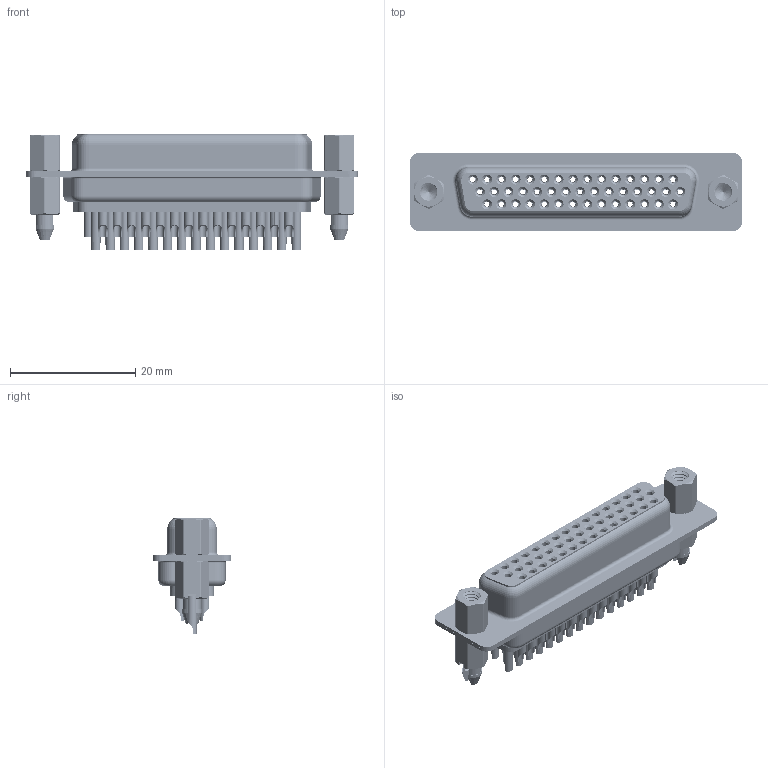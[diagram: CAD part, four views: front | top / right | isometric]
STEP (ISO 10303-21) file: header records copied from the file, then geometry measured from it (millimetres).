
FILE_DESCRIPTION (( 'STEP AP203' ), '1' );
FILE_NAME ('638-044-232-247.STEP', '2020-07-18T22:45:11', ( '' ), ( '' ), 'SwSTEP 2.0', 'SolidWorks 2020', '' );
FILE_SCHEMA (( 'CONFIG_CONTROL_DESIGN' ));
Length unit declared in the file: millimetre
Products named in the file (9): 638-044-232-247; 638 Shell Rear_44 Contacts; 638 Contact Row 1_32; 638 Shell Front_44 Contacts; 638 Contact Row 3_32; 638 Contact Row 2_32; 638 4-40 Threaded Boardlock_LP; 638 Housing_44 Contacts; 638 4-40 Hex Standoff
Assembly tree (51 placements, depth 2):
  638-044-232-247
    638 Housing_44 Contacts
    638 Shell Front_44 Contacts
    638 Shell Rear_44 Contacts
    638 Contact Row 1_32  x15
    638 Contact Row 2_32  x15
    638 Contact Row 3_32  x14
    638 4-40 Hex Standoff  x2
    638 4-40 Threaded Boardlock_LP  x2
Bounding box: 53.04 x 12.6 x 18.6 mm (x, y, z)
Volume: 3669.4 mm3; surface area: 14295.8 mm2
Topology: 51 solids, 51 shells, 4395 faces, 11209 edges, 7057 vertices
Faces by surface type: cylinder 1341, plane 1045, bspline 898, torus 849, cone 262
Entity records: 41891 total; most frequent: CARTESIAN_POINT 12969, DIRECTION 5859, ORIENTED_EDGE 5436, EDGE_CURVE 2718, AXIS2_PLACEMENT_3D 2452, VERTEX_POINT 1730, EDGE_LOOP 1390, CIRCLE 1321
